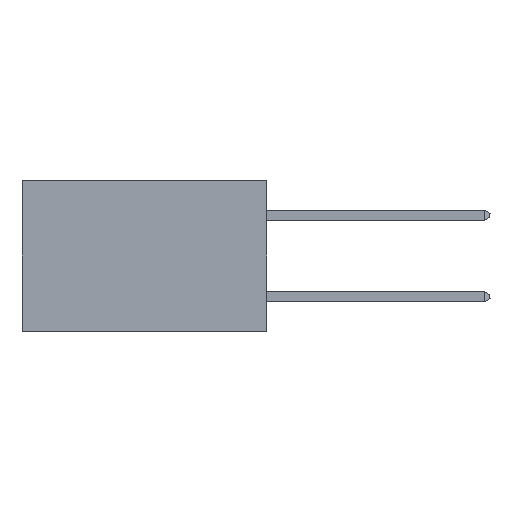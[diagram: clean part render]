
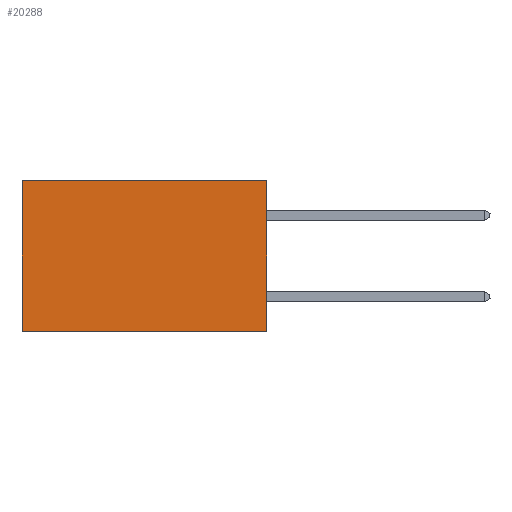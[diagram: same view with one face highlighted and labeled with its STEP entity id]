
A CAD part, left-side view. The second image highlights one B-rep face of the part: STEP entity #20288.
In plain terms, the highlighted planar face has unit normal (-1, 0, 0).
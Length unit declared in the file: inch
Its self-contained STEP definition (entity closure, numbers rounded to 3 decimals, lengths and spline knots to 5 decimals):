
#153 = VERTEX_POINT ( 'NONE', #2835 ) ;
#1132 = LINE ( 'NONE', #4476, #27226 ) ;
#1406 = CARTESIAN_POINT ( 'NONE',  ( 0.2875, 0., -0.37 ) ) ;
#1653 = CARTESIAN_POINT ( 'NONE',  ( 0.2875, 0., 0. ) ) ;
#2835 = CARTESIAN_POINT ( 'NONE',  ( 0.2875, 0.6, -0.37 ) ) ;
#2883 = CARTESIAN_POINT ( 'NONE',  ( 0.2875, 0., 0. ) ) ;
#4476 = CARTESIAN_POINT ( 'NONE',  ( 0.2875, 0.6, 0. ) ) ;
#7082 = VECTOR ( 'NONE', #29259, 39.37008 ) ;
#7214 = AXIS2_PLACEMENT_3D ( 'NONE', #18185, #20704, #30888 ) ;
#7263 = VERTEX_POINT ( 'NONE', #19812 ) ;
#8810 = ORIENTED_EDGE ( 'NONE', *, *, #25581, .F. ) ;
#9389 = CARTESIAN_POINT ( 'NONE',  ( 0.2875, 0., 0. ) ) ;
#12865 = EDGE_CURVE ( 'NONE', #17727, #28254, #28187, .T. ) ;
#13188 = FACE_OUTER_BOUND ( 'NONE', #14943, .T. ) ;
#13376 = LINE ( 'NONE', #9389, #13752 ) ;
#13752 = VECTOR ( 'NONE', #19412, 39.37008 ) ;
#14943 = EDGE_LOOP ( 'NONE', ( #15994, #8810, #18133, #19937 ) ) ;
#15994 = ORIENTED_EDGE ( 'NONE', *, *, #17841, .T. ) ;
#16204 = PLANE ( 'NONE',  #7214 ) ;
#17327 = DIRECTION ( 'NONE',  ( 0., 0., -1. ) ) ;
#17727 = VERTEX_POINT ( 'NONE', #2883 ) ;
#17841 = EDGE_CURVE ( 'NONE', #28254, #153, #1132, .T. ) ;
#17931 = EDGE_CURVE ( 'NONE', #17727, #7263, #13376, .T. ) ;
#18133 = ORIENTED_EDGE ( 'NONE', *, *, #17931, .F. ) ;
#18185 = CARTESIAN_POINT ( 'NONE',  ( 0.2875, 0., 0. ) ) ;
#18527 = LINE ( 'NONE', #1406, #7082 ) ;
#19412 = DIRECTION ( 'NONE',  ( 0., 0., -1. ) ) ;
#19812 = CARTESIAN_POINT ( 'NONE',  ( 0.2875, 0., -0.37 ) ) ;
#19885 = VECTOR ( 'NONE', #31704, 39.37008 ) ;
#19937 = ORIENTED_EDGE ( 'NONE', *, *, #12865, .T. ) ;
#20288 = ADVANCED_FACE ( 'NONE', ( #13188 ), #16204, .F. ) ;
#20704 = DIRECTION ( 'NONE',  ( 1., 0., 0. ) ) ;
#23508 = CARTESIAN_POINT ( 'NONE',  ( 0.2875, 0.6, 0. ) ) ;
#25581 = EDGE_CURVE ( 'NONE', #7263, #153, #18527, .T. ) ;
#27226 = VECTOR ( 'NONE', #17327, 39.37008 ) ;
#28187 = LINE ( 'NONE', #1653, #19885 ) ;
#28254 = VERTEX_POINT ( 'NONE', #23508 ) ;
#29259 = DIRECTION ( 'NONE',  ( 0., 1., 0. ) ) ;
#30888 = DIRECTION ( 'NONE',  ( 0., 0., -1. ) ) ;
#31704 = DIRECTION ( 'NONE',  ( 0., 1., 0. ) ) ;
